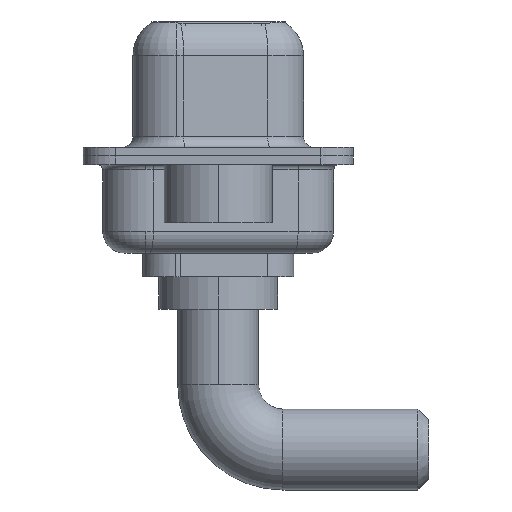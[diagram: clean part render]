
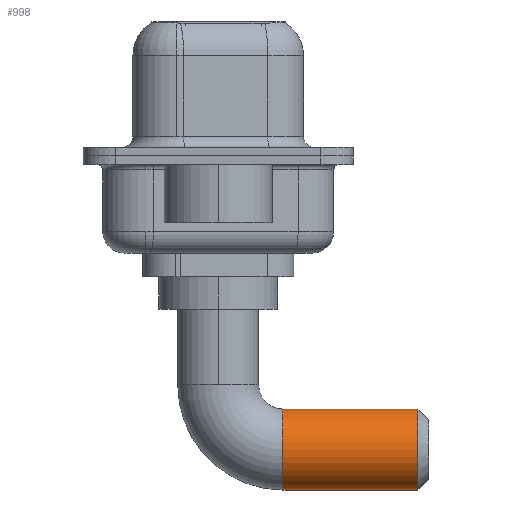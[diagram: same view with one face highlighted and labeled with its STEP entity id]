
A CAD part, left-side view. The second image highlights one B-rep face of the part: STEP entity #998.
In plain terms, the highlighted cylindrical face has radius 1.875 mm (diameter 3.75 mm), a partial arc.
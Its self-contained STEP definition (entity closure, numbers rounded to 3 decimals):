
#5 = DIRECTION ( 'NONE',  ( 0., -1., 0. ) ) ;
#604 = AXIS2_PLACEMENT_3D ( 'NONE', #7372, #7312, #8110 ) ;
#627 = ORIENTED_EDGE ( 'NONE', *, *, #5337, .T. ) ;
#998 = ADVANCED_FACE ( 'NONE', ( #7188 ), #6262, .T. ) ;
#1063 = EDGE_CURVE ( 'NONE', #7253, #11914, #2628, .T. ) ;
#1398 = VECTOR ( 'NONE', #2691, 1000. ) ;
#1723 = CARTESIAN_POINT ( 'NONE',  ( 0., -3., -6.5 ) ) ;
#2006 = VECTOR ( 'NONE', #12057, 1000. ) ;
#2460 = AXIS2_PLACEMENT_3D ( 'NONE', #5837, #9605, #8785 ) ;
#2628 = LINE ( 'NONE', #7251, #1398 ) ;
#2691 = DIRECTION ( 'NONE',  ( 0., -1., 0. ) ) ;
#2951 = CARTESIAN_POINT ( 'NONE',  ( 0., -9.25, -8.375 ) ) ;
#3453 = LINE ( 'NONE', #10191, #2006 ) ;
#4077 = AXIS2_PLACEMENT_3D ( 'NONE', #1723, #5, #9183 ) ;
#5224 = ORIENTED_EDGE ( 'NONE', *, *, #11470, .T. ) ;
#5337 = EDGE_CURVE ( 'NONE', #11016, #5509, #3453, .T. ) ;
#5509 = VERTEX_POINT ( 'NONE', #2951 ) ;
#5543 = ORIENTED_EDGE ( 'NONE', *, *, #1063, .F. ) ;
#5772 = CARTESIAN_POINT ( 'NONE',  ( 0., -3., -4.625 ) ) ;
#5837 = CARTESIAN_POINT ( 'NONE',  ( 0., -9.25, -6.5 ) ) ;
#6262 = CYLINDRICAL_SURFACE ( 'NONE', #604, 1.875 ) ;
#7188 = FACE_OUTER_BOUND ( 'NONE', #9474, .T. ) ;
#7251 = CARTESIAN_POINT ( 'NONE',  ( 0., -3., -4.625 ) ) ;
#7253 = VERTEX_POINT ( 'NONE', #5772 ) ;
#7312 = DIRECTION ( 'NONE',  ( 0., -1., 0. ) ) ;
#7372 = CARTESIAN_POINT ( 'NONE',  ( 0., -3., -6.5 ) ) ;
#7477 = EDGE_CURVE ( 'NONE', #5509, #11914, #7766, .T. ) ;
#7766 = CIRCLE ( 'NONE', #2460, 1.875 ) ;
#8110 = DIRECTION ( 'NONE',  ( 0., 0., -1. ) ) ;
#8785 = DIRECTION ( 'NONE',  ( 0., 0., -1. ) ) ;
#9183 = DIRECTION ( 'NONE',  ( -1., 0., 0. ) ) ;
#9289 = CARTESIAN_POINT ( 'NONE',  ( 0., -9.25, -4.625 ) ) ;
#9474 = EDGE_LOOP ( 'NONE', ( #5543, #5224, #627, #10936 ) ) ;
#9605 = DIRECTION ( 'NONE',  ( 0., 1., 0. ) ) ;
#10191 = CARTESIAN_POINT ( 'NONE',  ( 0., -3., -8.375 ) ) ;
#10936 = ORIENTED_EDGE ( 'NONE', *, *, #7477, .T. ) ;
#10989 = CIRCLE ( 'NONE', #4077, 1.875 ) ;
#11016 = VERTEX_POINT ( 'NONE', #11435 ) ;
#11435 = CARTESIAN_POINT ( 'NONE',  ( 0., -3., -8.375 ) ) ;
#11470 = EDGE_CURVE ( 'NONE', #7253, #11016, #10989, .T. ) ;
#11914 = VERTEX_POINT ( 'NONE', #9289 ) ;
#12057 = DIRECTION ( 'NONE',  ( 0., -1., 0. ) ) ;
